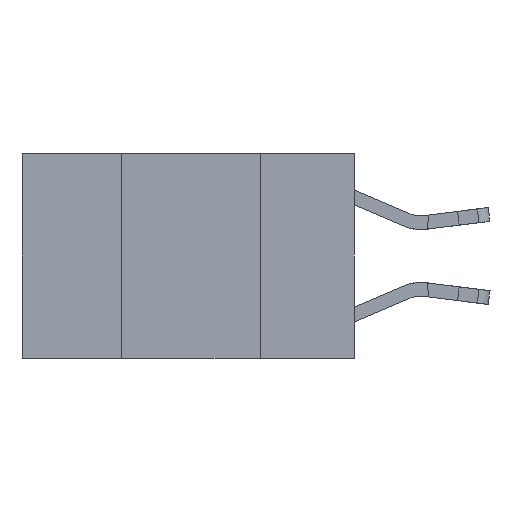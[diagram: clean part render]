
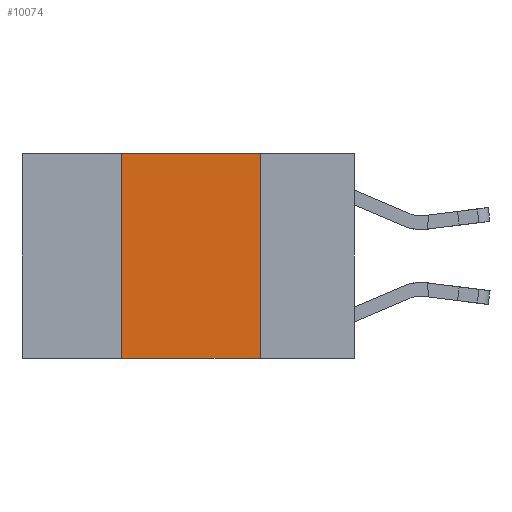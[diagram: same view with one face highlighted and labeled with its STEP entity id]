
A CAD part, left-side view. The second image highlights one B-rep face of the part: STEP entity #10074.
In plain terms, the highlighted planar face has unit normal (-1, 0, 0).
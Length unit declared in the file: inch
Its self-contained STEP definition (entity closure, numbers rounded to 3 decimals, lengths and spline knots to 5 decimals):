
#426 = LINE ( 'NONE', #7428, #8047 ) ;
#1996 = CARTESIAN_POINT ( 'NONE',  ( 0., 0.17, 0. ) ) ;
#2533 = AXIS2_PLACEMENT_3D ( 'NONE', #10245, #11750, #2642 ) ;
#2642 = DIRECTION ( 'NONE',  ( 0., 0., -1. ) ) ;
#3509 = ORIENTED_EDGE ( 'NONE', *, *, #10552, .T. ) ;
#3518 = VECTOR ( 'NONE', #5468, 39.37008 ) ;
#3769 = EDGE_CURVE ( 'NONE', #15174, #19501, #12718, .T. ) ;
#4435 = CARTESIAN_POINT ( 'NONE',  ( 0., 0.17, -0.37 ) ) ;
#4451 = DIRECTION ( 'NONE',  ( 0., -1., 0. ) ) ;
#4614 = VECTOR ( 'NONE', #15588, 39.37008 ) ;
#5156 = VECTOR ( 'NONE', #12647, 39.37008 ) ;
#5468 = DIRECTION ( 'NONE',  ( 0., -1., 0. ) ) ;
#7428 = CARTESIAN_POINT ( 'NONE',  ( 0., 0.6, 0. ) ) ;
#8030 = LINE ( 'NONE', #17580, #3518 ) ;
#8047 = VECTOR ( 'NONE', #4451, 39.37008 ) ;
#8111 = VERTEX_POINT ( 'NONE', #4435 ) ;
#8598 = CARTESIAN_POINT ( 'NONE',  ( 0., 0.42, 0. ) ) ;
#8635 = ORIENTED_EDGE ( 'NONE', *, *, #16505, .F. ) ;
#10074 = ADVANCED_FACE ( 'NONE', ( #19591 ), #19209, .F. ) ;
#10245 = CARTESIAN_POINT ( 'NONE',  ( 0., 0.6, 0. ) ) ;
#10552 = EDGE_CURVE ( 'NONE', #15174, #8111, #8030, .T. ) ;
#11302 = VERTEX_POINT ( 'NONE', #14216 ) ;
#11750 = DIRECTION ( 'NONE',  ( 1., 0., 0. ) ) ;
#12647 = DIRECTION ( 'NONE',  ( 0., 0., -1. ) ) ;
#12696 = ORIENTED_EDGE ( 'NONE', *, *, #3769, .F. ) ;
#12718 = LINE ( 'NONE', #16514, #4614 ) ;
#13234 = LINE ( 'NONE', #1996, #5156 ) ;
#14216 = CARTESIAN_POINT ( 'NONE',  ( 0., 0.17, 0. ) ) ;
#14886 = EDGE_CURVE ( 'NONE', #19501, #11302, #426, .T. ) ;
#15174 = VERTEX_POINT ( 'NONE', #18630 ) ;
#15499 = EDGE_LOOP ( 'NONE', ( #8635, #18766, #12696, #3509 ) ) ;
#15588 = DIRECTION ( 'NONE',  ( 0., 0., 1. ) ) ;
#16505 = EDGE_CURVE ( 'NONE', #11302, #8111, #13234, .T. ) ;
#16514 = CARTESIAN_POINT ( 'NONE',  ( 0., 0.42, 0. ) ) ;
#17580 = CARTESIAN_POINT ( 'NONE',  ( 0., 0.6, -0.37 ) ) ;
#18630 = CARTESIAN_POINT ( 'NONE',  ( 0., 0.42, -0.37 ) ) ;
#18766 = ORIENTED_EDGE ( 'NONE', *, *, #14886, .F. ) ;
#19209 = PLANE ( 'NONE',  #2533 ) ;
#19501 = VERTEX_POINT ( 'NONE', #8598 ) ;
#19591 = FACE_OUTER_BOUND ( 'NONE', #15499, .T. ) ;
